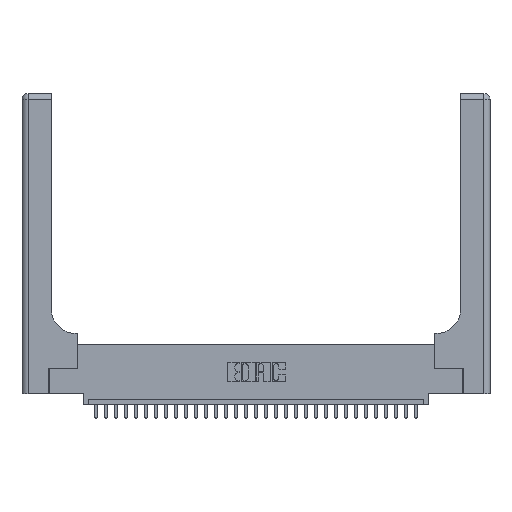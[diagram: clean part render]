
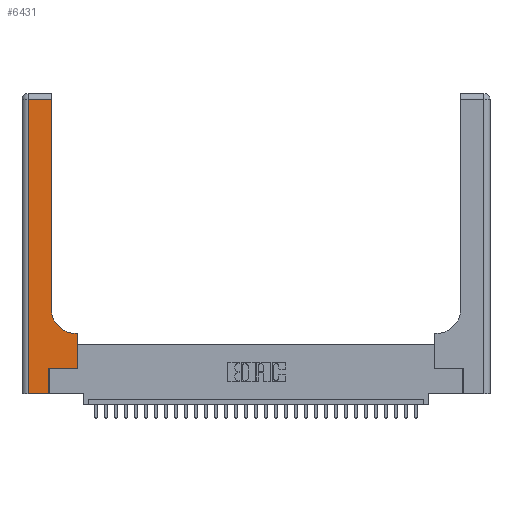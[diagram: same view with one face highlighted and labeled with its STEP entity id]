
A CAD part, top view. The second image highlights one B-rep face of the part: STEP entity #6431.
In plain terms, the highlighted planar face has unit normal (0, 0, 1).
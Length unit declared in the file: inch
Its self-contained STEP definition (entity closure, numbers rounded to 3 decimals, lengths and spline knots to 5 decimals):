
#379 = AXIS2_PLACEMENT_3D ( 'NONE', #16697, #11823, #23899 ) ;
#512 = VERTEX_POINT ( 'NONE', #26134 ) ;
#657 = CARTESIAN_POINT ( 'NONE',  ( 0.269, 0., 0.37 ) ) ;
#2035 = VECTOR ( 'NONE', #25368, 39.37008 ) ;
#3968 = ORIENTED_EDGE ( 'NONE', *, *, #27707, .T. ) ;
#4575 = CARTESIAN_POINT ( 'NONE',  ( 0.06, 3., 0.37 ) ) ;
#4700 = DIRECTION ( 'NONE',  ( 0., 0., -1. ) ) ;
#5119 = CIRCLE ( 'NONE', #379, 0.25 ) ;
#5183 = VECTOR ( 'NONE', #10300, 39.37008 ) ;
#5838 = ORIENTED_EDGE ( 'NONE', *, *, #9912, .T. ) ;
#6054 = LINE ( 'NONE', #4575, #9075 ) ;
#6239 = EDGE_CURVE ( 'NONE', #7192, #23383, #10282, .T. ) ;
#6431 = ADVANCED_FACE ( 'NONE', ( #27723 ), #19200, .F. ) ;
#6946 = LINE ( 'NONE', #20275, #2035 ) ;
#7142 = DIRECTION ( 'NONE',  ( -1., 0., 0. ) ) ;
#7192 = VERTEX_POINT ( 'NONE', #30837 ) ;
#7273 = CARTESIAN_POINT ( 'NONE',  ( 0.5585, 0.25, 0.37 ) ) ;
#8236 = LINE ( 'NONE', #657, #5183 ) ;
#8322 = DIRECTION ( 'NONE',  ( -1., 0., 0. ) ) ;
#9033 = ORIENTED_EDGE ( 'NONE', *, *, #22415, .T. ) ;
#9075 = VECTOR ( 'NONE', #23940, 39.37008 ) ;
#9698 = DIRECTION ( 'NONE',  ( -1., 0., 0. ) ) ;
#9912 = EDGE_CURVE ( 'NONE', #512, #26067, #5119, .T. ) ;
#10134 = VECTOR ( 'NONE', #8322, 39.37008 ) ;
#10282 = LINE ( 'NONE', #7273, #20865 ) ;
#10300 = DIRECTION ( 'NONE',  ( 0., 1., 0. ) ) ;
#11596 = EDGE_CURVE ( 'NONE', #26067, #19035, #6946, .T. ) ;
#11713 = VECTOR ( 'NONE', #27799, 39.37008 ) ;
#11823 = DIRECTION ( 'NONE',  ( 0., 0., -1. ) ) ;
#12317 = VECTOR ( 'NONE', #9698, 39.37008 ) ;
#12503 = VECTOR ( 'NONE', #18074, 39.37008 ) ;
#12666 = ORIENTED_EDGE ( 'NONE', *, *, #31141, .T. ) ;
#13076 = CARTESIAN_POINT ( 'NONE',  ( 0.5585, 0.6, 0.37 ) ) ;
#13210 = CARTESIAN_POINT ( 'NONE',  ( 0., 0., 0.37 ) ) ;
#14638 = ORIENTED_EDGE ( 'NONE', *, *, #11596, .T. ) ;
#14711 = ORIENTED_EDGE ( 'NONE', *, *, #26261, .T. ) ;
#15034 = LINE ( 'NONE', #18045, #10134 ) ;
#15119 = CARTESIAN_POINT ( 'NONE',  ( 0.2915, 2.94, 0.37 ) ) ;
#15949 = CARTESIAN_POINT ( 'NONE',  ( 0.06, 2.94, 0.37 ) ) ;
#16697 = CARTESIAN_POINT ( 'NONE',  ( 0.5415, 0.85, 0.37 ) ) ;
#17318 = DIRECTION ( 'NONE',  ( 0., 1., 0. ) ) ;
#17521 = ORIENTED_EDGE ( 'NONE', *, *, #26731, .T. ) ;
#17717 = ORIENTED_EDGE ( 'NONE', *, *, #22910, .T. ) ;
#18045 = CARTESIAN_POINT ( 'NONE',  ( 0., 2.94, 0.37 ) ) ;
#18074 = DIRECTION ( 'NONE',  ( 1., 0., 0. ) ) ;
#18148 = LINE ( 'NONE', #25257, #11713 ) ;
#18300 = ORIENTED_EDGE ( 'NONE', *, *, #6239, .T. ) ;
#18944 = LINE ( 'NONE', #13210, #12503 ) ;
#19035 = VERTEX_POINT ( 'NONE', #15119 ) ;
#19098 = CARTESIAN_POINT ( 'NONE',  ( 0., 3., 0.37 ) ) ;
#19200 = PLANE ( 'NONE',  #22213 ) ;
#19331 = CARTESIAN_POINT ( 'NONE',  ( 0.269, 0.25, 0.37 ) ) ;
#20275 = CARTESIAN_POINT ( 'NONE',  ( 0.2915, 3., 0.37 ) ) ;
#20830 = VERTEX_POINT ( 'NONE', #19331 ) ;
#20865 = VECTOR ( 'NONE', #17318, 39.37008 ) ;
#21220 = CARTESIAN_POINT ( 'NONE',  ( 0.2915, 0.85, 0.37 ) ) ;
#21512 = EDGE_LOOP ( 'NONE', ( #14638, #14711, #12666, #9033, #17521, #17717, #18300, #3968, #5838 ) ) ;
#21540 = CARTESIAN_POINT ( 'NONE',  ( 0.2915, 0.6, 0.37 ) ) ;
#22213 = AXIS2_PLACEMENT_3D ( 'NONE', #19098, #4700, #7142 ) ;
#22415 = EDGE_CURVE ( 'NONE', #26004, #24626, #18944, .T. ) ;
#22910 = EDGE_CURVE ( 'NONE', #20830, #7192, #18148, .T. ) ;
#23383 = VERTEX_POINT ( 'NONE', #13076 ) ;
#23899 = DIRECTION ( 'NONE',  ( 1., 0., 0. ) ) ;
#23940 = DIRECTION ( 'NONE',  ( 0., -1., 0. ) ) ;
#24626 = VERTEX_POINT ( 'NONE', #25613 ) ;
#25257 = CARTESIAN_POINT ( 'NONE',  ( 0.269, 0.25, 0.37 ) ) ;
#25368 = DIRECTION ( 'NONE',  ( 0., 1., 0. ) ) ;
#25613 = CARTESIAN_POINT ( 'NONE',  ( 0.269, 0., 0.37 ) ) ;
#25998 = CARTESIAN_POINT ( 'NONE',  ( 0.06, 0., 0.37 ) ) ;
#26004 = VERTEX_POINT ( 'NONE', #25998 ) ;
#26067 = VERTEX_POINT ( 'NONE', #21220 ) ;
#26134 = CARTESIAN_POINT ( 'NONE',  ( 0.5415, 0.6, 0.37 ) ) ;
#26261 = EDGE_CURVE ( 'NONE', #19035, #27518, #15034, .T. ) ;
#26731 = EDGE_CURVE ( 'NONE', #24626, #20830, #8236, .T. ) ;
#27518 = VERTEX_POINT ( 'NONE', #15949 ) ;
#27707 = EDGE_CURVE ( 'NONE', #23383, #512, #30927, .T. ) ;
#27723 = FACE_OUTER_BOUND ( 'NONE', #21512, .T. ) ;
#27799 = DIRECTION ( 'NONE',  ( 1., 0., 0. ) ) ;
#30837 = CARTESIAN_POINT ( 'NONE',  ( 0.5585, 0.25, 0.37 ) ) ;
#30927 = LINE ( 'NONE', #21540, #12317 ) ;
#31141 = EDGE_CURVE ( 'NONE', #27518, #26004, #6054, .T. ) ;
